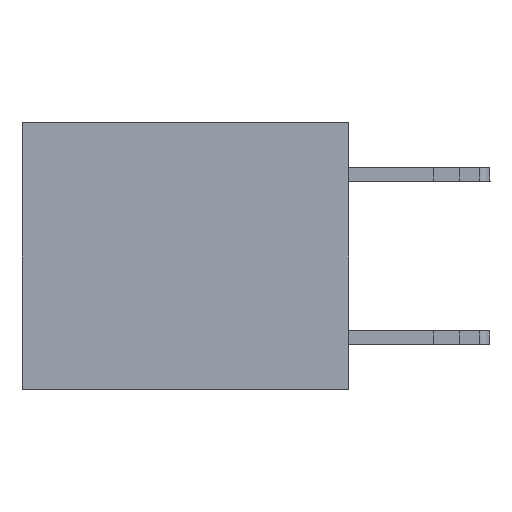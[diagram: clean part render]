
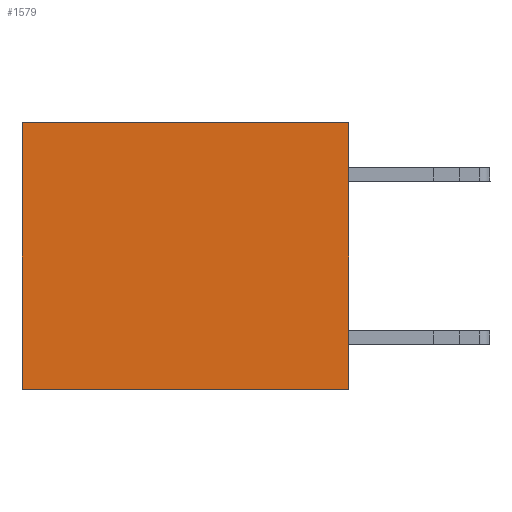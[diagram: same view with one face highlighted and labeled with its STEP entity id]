
A CAD part, left-side view. The second image highlights one B-rep face of the part: STEP entity #1579.
In plain terms, the highlighted planar face has unit normal (-1, 0, 0).
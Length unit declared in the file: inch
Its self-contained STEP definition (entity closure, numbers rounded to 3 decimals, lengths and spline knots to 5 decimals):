
#267 = EDGE_CURVE ( 'NONE', #21267, #1701, #7567, .T. ) ;
#1579 = ADVANCED_FACE ( 'NONE', ( #9297 ), #12851, .F. ) ;
#1701 = VERTEX_POINT ( 'NONE', #5925 ) ;
#3168 = VECTOR ( 'NONE', #5955, 39.37008 ) ;
#3181 = DIRECTION ( 'NONE',  ( 0., 0., -1. ) ) ;
#3731 = ORIENTED_EDGE ( 'NONE', *, *, #19983, .F. ) ;
#3950 = CARTESIAN_POINT ( 'NONE',  ( 0.3165, 0.6, -0.49 ) ) ;
#5860 = LINE ( 'NONE', #24996, #16688 ) ;
#5925 = CARTESIAN_POINT ( 'NONE',  ( 0.3165, 0.6, 0. ) ) ;
#5955 = DIRECTION ( 'NONE',  ( 0., 1., 0. ) ) ;
#7567 = LINE ( 'NONE', #11947, #3168 ) ;
#8266 = EDGE_CURVE ( 'NONE', #13062, #9252, #5860, .T. ) ;
#8630 = ORIENTED_EDGE ( 'NONE', *, *, #21836, .T. ) ;
#8655 = LINE ( 'NONE', #11103, #18571 ) ;
#9252 = VERTEX_POINT ( 'NONE', #3950 ) ;
#9297 = FACE_OUTER_BOUND ( 'NONE', #16563, .T. ) ;
#11103 = CARTESIAN_POINT ( 'NONE',  ( 0.3165, 0., -0.49 ) ) ;
#11143 = DIRECTION ( 'NONE',  ( 0., 0., -1. ) ) ;
#11554 = DIRECTION ( 'NONE',  ( 0., 0., -1. ) ) ;
#11947 = CARTESIAN_POINT ( 'NONE',  ( 0.3165, 0., 0. ) ) ;
#12455 = CARTESIAN_POINT ( 'NONE',  ( 0.3165, 0., -0.49 ) ) ;
#12851 = PLANE ( 'NONE',  #17127 ) ;
#12858 = ORIENTED_EDGE ( 'NONE', *, *, #267, .T. ) ;
#13062 = VERTEX_POINT ( 'NONE', #22598 ) ;
#13541 = VECTOR ( 'NONE', #11554, 39.37008 ) ;
#15856 = DIRECTION ( 'NONE',  ( 1., 0., 0. ) ) ;
#16563 = EDGE_LOOP ( 'NONE', ( #8630, #25115, #3731, #12858 ) ) ;
#16688 = VECTOR ( 'NONE', #22484, 39.37008 ) ;
#17127 = AXIS2_PLACEMENT_3D ( 'NONE', #12455, #15856, #11143 ) ;
#18142 = LINE ( 'NONE', #21313, #13541 ) ;
#18571 = VECTOR ( 'NONE', #3181, 39.37008 ) ;
#19983 = EDGE_CURVE ( 'NONE', #21267, #13062, #8655, .T. ) ;
#21267 = VERTEX_POINT ( 'NONE', #22738 ) ;
#21313 = CARTESIAN_POINT ( 'NONE',  ( 0.3165, 0.6, -0.49 ) ) ;
#21836 = EDGE_CURVE ( 'NONE', #1701, #9252, #18142, .T. ) ;
#22484 = DIRECTION ( 'NONE',  ( 0., 1., 0. ) ) ;
#22598 = CARTESIAN_POINT ( 'NONE',  ( 0.3165, 0., -0.49 ) ) ;
#22738 = CARTESIAN_POINT ( 'NONE',  ( 0.3165, 0., 0. ) ) ;
#24996 = CARTESIAN_POINT ( 'NONE',  ( 0.3165, 0., -0.49 ) ) ;
#25115 = ORIENTED_EDGE ( 'NONE', *, *, #8266, .F. ) ;
